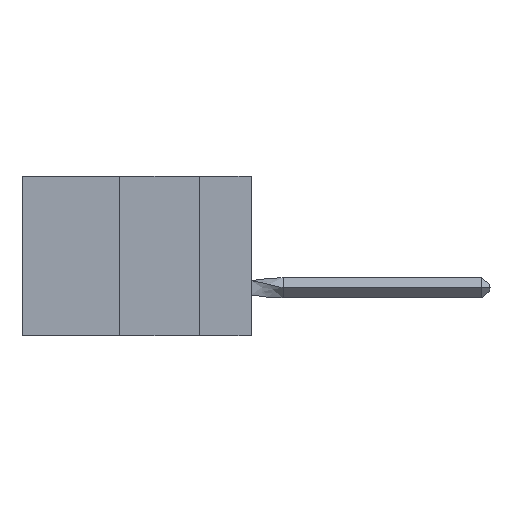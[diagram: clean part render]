
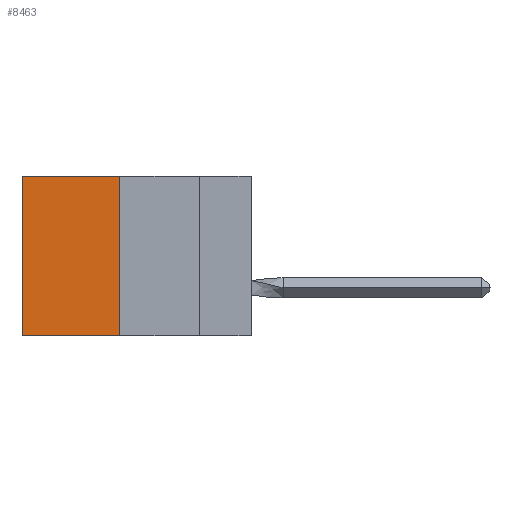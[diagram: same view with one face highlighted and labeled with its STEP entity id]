
A CAD part, left-side view. The second image highlights one B-rep face of the part: STEP entity #8463.
In plain terms, the highlighted planar face has unit normal (-1, 0, 0).
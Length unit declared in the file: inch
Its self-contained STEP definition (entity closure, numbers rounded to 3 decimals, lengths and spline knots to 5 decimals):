
#17 = CARTESIAN_POINT ( 'NONE',  ( 0.305, 0.413, 0. ) ) ;
#181 = VECTOR ( 'NONE', #783, 39.37008 ) ;
#607 = EDGE_LOOP ( 'NONE', ( #6231, #9284, #5557, #8254 ) ) ;
#783 = DIRECTION ( 'NONE',  ( 0., 0., -1. ) ) ;
#1565 = VECTOR ( 'NONE', #11791, 39.37008 ) ;
#1574 = EDGE_CURVE ( 'NONE', #13799, #8346, #14665, .T. ) ;
#1853 = LINE ( 'NONE', #17, #14602 ) ;
#1885 = CARTESIAN_POINT ( 'NONE',  ( 0.305, 0.413, -0.5 ) ) ;
#2609 = LINE ( 'NONE', #11154, #11415 ) ;
#3533 = DIRECTION ( 'NONE',  ( 0., 1., 0. ) ) ;
#4374 = PLANE ( 'NONE',  #11457 ) ;
#4643 = DIRECTION ( 'NONE',  ( 0., 0., -1. ) ) ;
#5358 = EDGE_CURVE ( 'NONE', #10727, #15230, #2609, .T. ) ;
#5500 = CARTESIAN_POINT ( 'NONE',  ( 0.305, 0.413, -0.5 ) ) ;
#5557 = ORIENTED_EDGE ( 'NONE', *, *, #5358, .F. ) ;
#6231 = ORIENTED_EDGE ( 'NONE', *, *, #1574, .T. ) ;
#6300 = CARTESIAN_POINT ( 'NONE',  ( 0.305, 0.413, -0.5 ) ) ;
#8254 = ORIENTED_EDGE ( 'NONE', *, *, #8728, .T. ) ;
#8346 = VERTEX_POINT ( 'NONE', #9478 ) ;
#8463 = ADVANCED_FACE ( 'NONE', ( #11706 ), #4374, .F. ) ;
#8645 = CARTESIAN_POINT ( 'NONE',  ( 0.305, 0.72, 0. ) ) ;
#8728 = EDGE_CURVE ( 'NONE', #10727, #13799, #1853, .T. ) ;
#9066 = LINE ( 'NONE', #5500, #1565 ) ;
#9284 = ORIENTED_EDGE ( 'NONE', *, *, #15844, .F. ) ;
#9432 = CARTESIAN_POINT ( 'NONE',  ( 0.305, 0.72, -0.5 ) ) ;
#9478 = CARTESIAN_POINT ( 'NONE',  ( 0.305, 0.72, -0.5 ) ) ;
#9946 = DIRECTION ( 'NONE',  ( 0., 0., -1. ) ) ;
#10727 = VERTEX_POINT ( 'NONE', #13061 ) ;
#11154 = CARTESIAN_POINT ( 'NONE',  ( 0.305, 0.413, -0.5 ) ) ;
#11415 = VECTOR ( 'NONE', #9946, 39.37008 ) ;
#11457 = AXIS2_PLACEMENT_3D ( 'NONE', #1885, #14430, #4643 ) ;
#11706 = FACE_OUTER_BOUND ( 'NONE', #607, .T. ) ;
#11791 = DIRECTION ( 'NONE',  ( 0., 1., 0. ) ) ;
#13061 = CARTESIAN_POINT ( 'NONE',  ( 0.305, 0.413, 0. ) ) ;
#13799 = VERTEX_POINT ( 'NONE', #8645 ) ;
#14430 = DIRECTION ( 'NONE',  ( 1., 0., 0. ) ) ;
#14602 = VECTOR ( 'NONE', #3533, 39.37008 ) ;
#14665 = LINE ( 'NONE', #9432, #181 ) ;
#15230 = VERTEX_POINT ( 'NONE', #6300 ) ;
#15844 = EDGE_CURVE ( 'NONE', #15230, #8346, #9066, .T. ) ;
